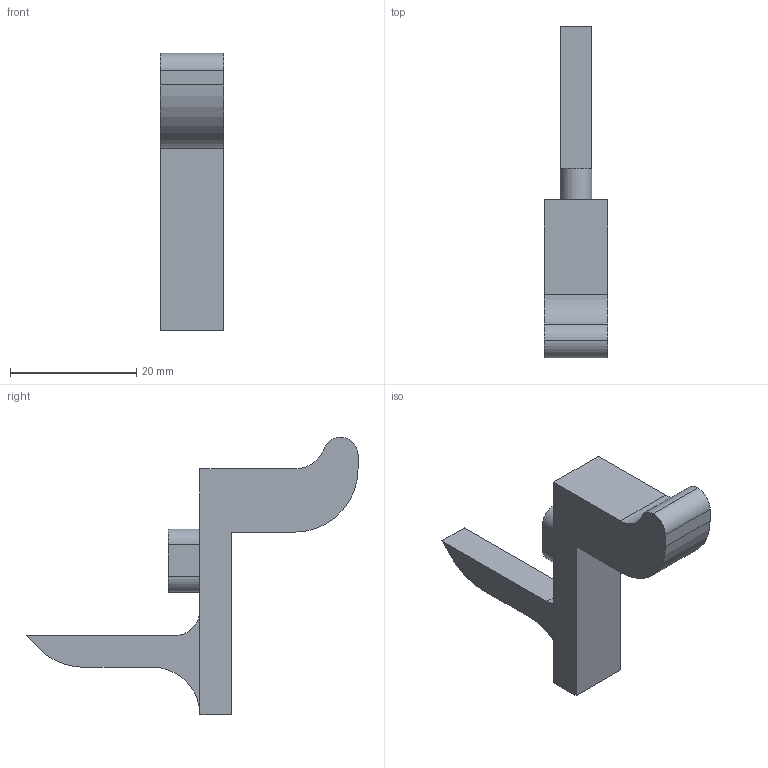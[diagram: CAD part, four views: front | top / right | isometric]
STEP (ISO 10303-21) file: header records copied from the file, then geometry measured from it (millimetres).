
FILE_DESCRIPTION (( 'STEP AP203' ), '1' );
FILE_NAME ('Trigger.STEP', '2013-08-28T12:44:47', ( '' ), ( '' ), 'SwSTEP 2.0', 'SolidWorks 2013', '' );
FILE_SCHEMA (( 'CONFIG_CONTROL_DESIGN' ));
Length unit declared in the file: millimetre
Products named in the file (1): Trigger
Bounding box: 10 x 52.5 x 43.86 mm (x, y, z)
Volume: 4922.4 mm3; surface area: 2734 mm2
Topology: 1 solids, 1 shells, 27 faces, 70 edges, 46 vertices
Faces by surface type: plane 17, cylinder 10
Entity records: 907 total; most frequent: DIRECTION 146, CARTESIAN_POINT 144, ORIENTED_EDGE 140, EDGE_CURVE 70, VECTOR 50, LINE 50, AXIS2_PLACEMENT_3D 48, VERTEX_POINT 46
